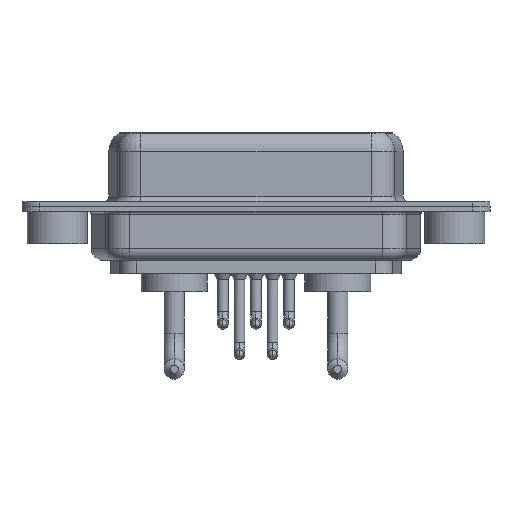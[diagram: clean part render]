
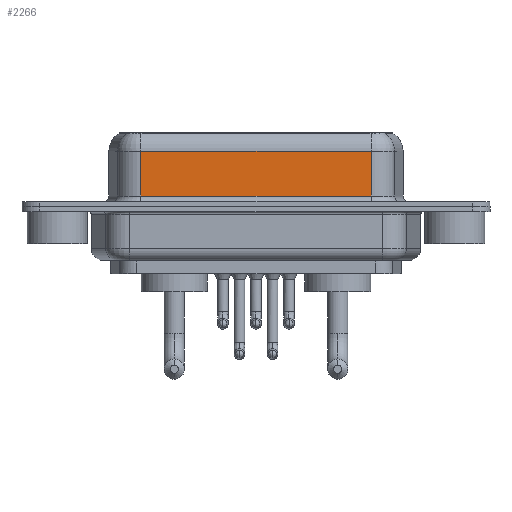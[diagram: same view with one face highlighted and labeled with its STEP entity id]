
A CAD part, front view. The second image highlights one B-rep face of the part: STEP entity #2266.
In plain terms, the highlighted planar face has unit normal (0, -1, 0).
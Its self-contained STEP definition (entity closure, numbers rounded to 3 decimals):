
#223 = LINE ( 'NONE', #4046, #11808 ) ;
#302 = VERTEX_POINT ( 'NONE', #6746 ) ;
#453 = ORIENTED_EDGE ( 'NONE', *, *, #12451, .F. ) ;
#1324 = DIRECTION ( 'NONE',  ( 0., 0., -1. ) ) ;
#1747 = EDGE_LOOP ( 'NONE', ( #453, #8265, #10973, #8023 ) ) ;
#2266 = ADVANCED_FACE ( 'NONE', ( #9001 ), #6258, .F. ) ;
#2277 = CARTESIAN_POINT ( 'NONE',  ( 7.013, -3.95, 6.4 ) ) ;
#2919 = CARTESIAN_POINT ( 'NONE',  ( 7.013, -3.95, 0.9 ) ) ;
#3941 = DIRECTION ( 'NONE',  ( 0., 0., 1. ) ) ;
#4017 = CARTESIAN_POINT ( 'NONE',  ( 26.287, -3.95, 4.65 ) ) ;
#4046 = CARTESIAN_POINT ( 'NONE',  ( 26.287, -3.95, 4.65 ) ) ;
#4382 = LINE ( 'NONE', #11133, #4890 ) ;
#4890 = VECTOR ( 'NONE', #16043, 1000. ) ;
#5136 = VECTOR ( 'NONE', #10543, 1000. ) ;
#5158 = LINE ( 'NONE', #14322, #5136 ) ;
#6174 = EDGE_CURVE ( 'NONE', #15821, #302, #223, .T. ) ;
#6258 = PLANE ( 'NONE',  #10592 ) ;
#6371 = CARTESIAN_POINT ( 'NONE',  ( 26.287, -3.95, 0.9 ) ) ;
#6746 = CARTESIAN_POINT ( 'NONE',  ( 7.013, -3.95, 4.65 ) ) ;
#8023 = ORIENTED_EDGE ( 'NONE', *, *, #13129, .T. ) ;
#8225 = VECTOR ( 'NONE', #1324, 1000. ) ;
#8265 = ORIENTED_EDGE ( 'NONE', *, *, #6174, .T. ) ;
#9001 = FACE_OUTER_BOUND ( 'NONE', #1747, .T. ) ;
#10477 = DIRECTION ( 'NONE',  ( -1., 0., 0. ) ) ;
#10543 = DIRECTION ( 'NONE',  ( 0., 0., -1. ) ) ;
#10592 = AXIS2_PLACEMENT_3D ( 'NONE', #15686, #16710, #3941 ) ;
#10973 = ORIENTED_EDGE ( 'NONE', *, *, #16736, .T. ) ;
#11133 = CARTESIAN_POINT ( 'NONE',  ( 26.287, -3.95, 0.9 ) ) ;
#11808 = VECTOR ( 'NONE', #10477, 1000. ) ;
#11867 = VERTEX_POINT ( 'NONE', #6371 ) ;
#12451 = EDGE_CURVE ( 'NONE', #15821, #11867, #5158, .T. ) ;
#13129 = EDGE_CURVE ( 'NONE', #13412, #11867, #4382, .T. ) ;
#13412 = VERTEX_POINT ( 'NONE', #2919 ) ;
#14322 = CARTESIAN_POINT ( 'NONE',  ( 26.287, -3.95, 6.4 ) ) ;
#15384 = LINE ( 'NONE', #2277, #8225 ) ;
#15686 = CARTESIAN_POINT ( 'NONE',  ( 26.287, -3.95, 6.4 ) ) ;
#15821 = VERTEX_POINT ( 'NONE', #4017 ) ;
#16043 = DIRECTION ( 'NONE',  ( 1., 0., 0. ) ) ;
#16710 = DIRECTION ( 'NONE',  ( 0., 1., 0. ) ) ;
#16736 = EDGE_CURVE ( 'NONE', #302, #13412, #15384, .T. ) ;
